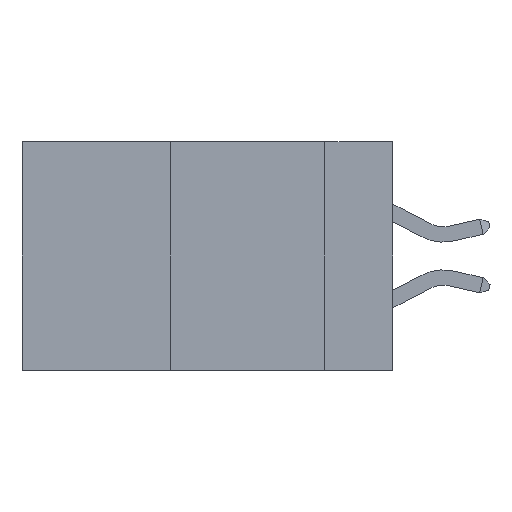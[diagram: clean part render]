
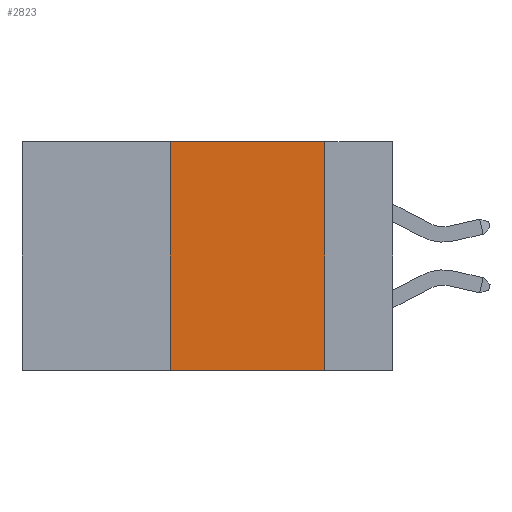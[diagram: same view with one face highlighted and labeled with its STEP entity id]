
A CAD part, left-side view. The second image highlights one B-rep face of the part: STEP entity #2823.
In plain terms, the highlighted planar face has unit normal (-1, 0, 0).
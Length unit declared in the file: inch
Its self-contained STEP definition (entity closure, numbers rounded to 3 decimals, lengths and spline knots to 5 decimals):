
#174 = DIRECTION ( 'NONE',  ( 0., 0., -1. ) ) ;
#332 = CARTESIAN_POINT ( 'NONE',  ( 0., 0.11, -0.37 ) ) ;
#720 = EDGE_LOOP ( 'NONE', ( #14250, #880, #10359, #17387 ) ) ;
#880 = ORIENTED_EDGE ( 'NONE', *, *, #21277, .F. ) ;
#1135 = VECTOR ( 'NONE', #5621, 39.37008 ) ;
#1142 = LINE ( 'NONE', #23248, #17669 ) ;
#1732 = CARTESIAN_POINT ( 'NONE',  ( 0., 0.6, 0. ) ) ;
#2266 = EDGE_CURVE ( 'NONE', #7746, #12224, #24267, .T. ) ;
#2496 = DIRECTION ( 'NONE',  ( 0., -1., 0. ) ) ;
#2823 = ADVANCED_FACE ( 'NONE', ( #20943 ), #20822, .F. ) ;
#5598 = VECTOR ( 'NONE', #18740, 39.37008 ) ;
#5621 = DIRECTION ( 'NONE',  ( 0., 0., 1. ) ) ;
#7746 = VERTEX_POINT ( 'NONE', #16296 ) ;
#8965 = LINE ( 'NONE', #27261, #5598 ) ;
#10359 = ORIENTED_EDGE ( 'NONE', *, *, #2266, .F. ) ;
#11899 = EDGE_CURVE ( 'NONE', #7746, #22093, #8965, .T. ) ;
#12224 = VERTEX_POINT ( 'NONE', #17632 ) ;
#14250 = ORIENTED_EDGE ( 'NONE', *, *, #19486, .F. ) ;
#14454 = DIRECTION ( 'NONE',  ( 0., 0., -1. ) ) ;
#15457 = VECTOR ( 'NONE', #174, 39.37008 ) ;
#16296 = CARTESIAN_POINT ( 'NONE',  ( 0., 0.36, -0.37 ) ) ;
#17387 = ORIENTED_EDGE ( 'NONE', *, *, #11899, .T. ) ;
#17632 = CARTESIAN_POINT ( 'NONE',  ( 0., 0.36, 0. ) ) ;
#17669 = VECTOR ( 'NONE', #2496, 39.37008 ) ;
#17806 = CARTESIAN_POINT ( 'NONE',  ( 0., 0.11, 0. ) ) ;
#18740 = DIRECTION ( 'NONE',  ( 0., -1., 0. ) ) ;
#19486 = EDGE_CURVE ( 'NONE', #23367, #22093, #21047, .T. ) ;
#19867 = AXIS2_PLACEMENT_3D ( 'NONE', #1732, #26628, #14454 ) ;
#20822 = PLANE ( 'NONE',  #19867 ) ;
#20943 = FACE_OUTER_BOUND ( 'NONE', #720, .T. ) ;
#21047 = LINE ( 'NONE', #23332, #15457 ) ;
#21277 = EDGE_CURVE ( 'NONE', #12224, #23367, #1142, .T. ) ;
#22093 = VERTEX_POINT ( 'NONE', #332 ) ;
#23248 = CARTESIAN_POINT ( 'NONE',  ( 0., 0.6, 0. ) ) ;
#23332 = CARTESIAN_POINT ( 'NONE',  ( 0., 0.11, 0. ) ) ;
#23367 = VERTEX_POINT ( 'NONE', #17806 ) ;
#24267 = LINE ( 'NONE', #24398, #1135 ) ;
#24398 = CARTESIAN_POINT ( 'NONE',  ( 0., 0.36, 0. ) ) ;
#26628 = DIRECTION ( 'NONE',  ( 1., 0., 0. ) ) ;
#27261 = CARTESIAN_POINT ( 'NONE',  ( 0., 0.6, -0.37 ) ) ;
